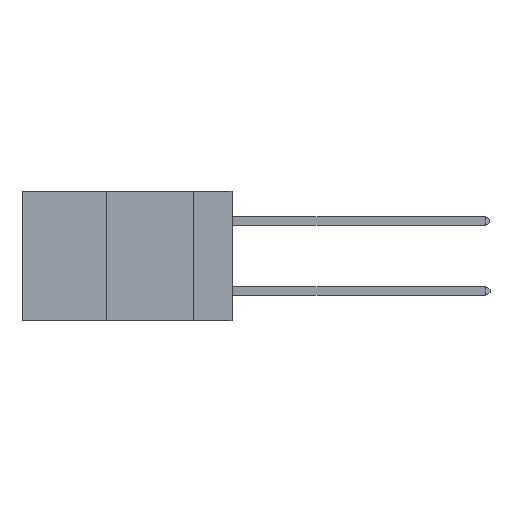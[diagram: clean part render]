
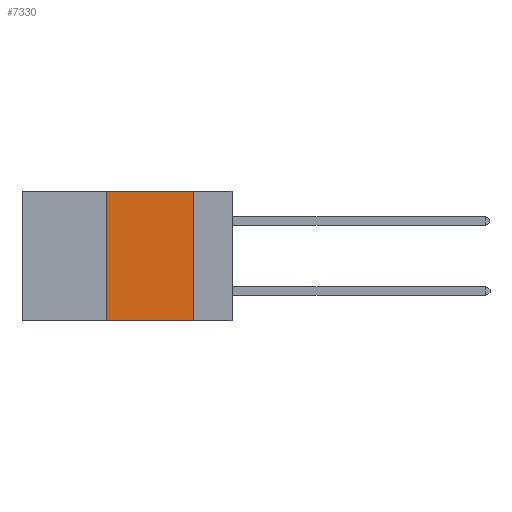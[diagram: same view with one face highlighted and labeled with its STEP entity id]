
A CAD part, left-side view. The second image highlights one B-rep face of the part: STEP entity #7330.
In plain terms, the highlighted planar face has unit normal (-1, 0, 0).
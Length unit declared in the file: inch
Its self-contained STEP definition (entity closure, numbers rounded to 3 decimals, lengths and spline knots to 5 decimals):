
#141 = CARTESIAN_POINT ( 'NONE',  ( 0., 0.6, 0. ) ) ;
#1058 = CARTESIAN_POINT ( 'NONE',  ( 0., 0.11, 0. ) ) ;
#1302 = VERTEX_POINT ( 'NONE', #19885 ) ;
#1534 = EDGE_CURVE ( 'NONE', #11235, #5218, #14501, .T. ) ;
#2017 = DIRECTION ( 'NONE',  ( 1., 0., 0. ) ) ;
#4873 = ORIENTED_EDGE ( 'NONE', *, *, #13834, .T. ) ;
#5042 = EDGE_CURVE ( 'NONE', #1302, #11235, #8153, .T. ) ;
#5218 = VERTEX_POINT ( 'NONE', #1058 ) ;
#5234 = CARTESIAN_POINT ( 'NONE',  ( 0., 0.36, 0. ) ) ;
#5716 = VECTOR ( 'NONE', #17974, 39.37008 ) ;
#7330 = ADVANCED_FACE ( 'NONE', ( #14706 ), #10970, .F. ) ;
#7418 = EDGE_CURVE ( 'NONE', #5218, #22596, #13029, .T. ) ;
#8153 = LINE ( 'NONE', #5234, #22827 ) ;
#8833 = DIRECTION ( 'NONE',  ( 0., 0., 1. ) ) ;
#10067 = EDGE_LOOP ( 'NONE', ( #13233, #22631, #18522, #4873 ) ) ;
#10970 = PLANE ( 'NONE',  #21544 ) ;
#11196 = DIRECTION ( 'NONE',  ( 0., 0., -1. ) ) ;
#11235 = VERTEX_POINT ( 'NONE', #19550 ) ;
#13029 = LINE ( 'NONE', #21838, #17766 ) ;
#13233 = ORIENTED_EDGE ( 'NONE', *, *, #7418, .F. ) ;
#13834 = EDGE_CURVE ( 'NONE', #1302, #22596, #19364, .T. ) ;
#14358 = CARTESIAN_POINT ( 'NONE',  ( 0., 0.6, 0. ) ) ;
#14374 = DIRECTION ( 'NONE',  ( 0., -1., 0. ) ) ;
#14501 = LINE ( 'NONE', #14358, #18687 ) ;
#14525 = DIRECTION ( 'NONE',  ( 0., 0., -1. ) ) ;
#14706 = FACE_OUTER_BOUND ( 'NONE', #10067, .T. ) ;
#15450 = CARTESIAN_POINT ( 'NONE',  ( 0., 0.11, -0.37 ) ) ;
#17766 = VECTOR ( 'NONE', #11196, 39.37008 ) ;
#17974 = DIRECTION ( 'NONE',  ( 0., -1., 0. ) ) ;
#18522 = ORIENTED_EDGE ( 'NONE', *, *, #5042, .F. ) ;
#18687 = VECTOR ( 'NONE', #14374, 39.37008 ) ;
#19364 = LINE ( 'NONE', #21484, #5716 ) ;
#19550 = CARTESIAN_POINT ( 'NONE',  ( 0., 0.36, 0. ) ) ;
#19885 = CARTESIAN_POINT ( 'NONE',  ( 0., 0.36, -0.37 ) ) ;
#21484 = CARTESIAN_POINT ( 'NONE',  ( 0., 0.6, -0.37 ) ) ;
#21544 = AXIS2_PLACEMENT_3D ( 'NONE', #141, #2017, #14525 ) ;
#21838 = CARTESIAN_POINT ( 'NONE',  ( 0., 0.11, 0. ) ) ;
#22596 = VERTEX_POINT ( 'NONE', #15450 ) ;
#22631 = ORIENTED_EDGE ( 'NONE', *, *, #1534, .F. ) ;
#22827 = VECTOR ( 'NONE', #8833, 39.37008 ) ;
